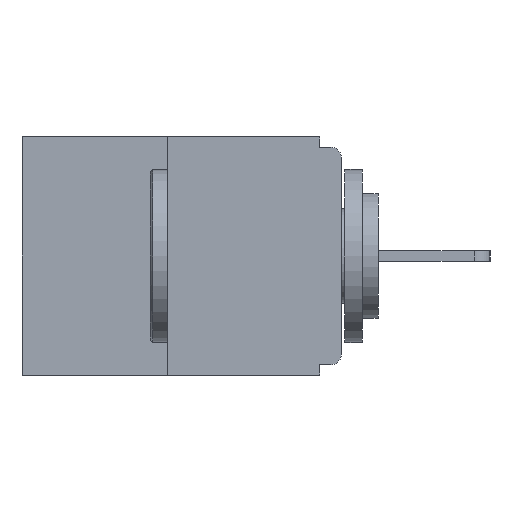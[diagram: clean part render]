
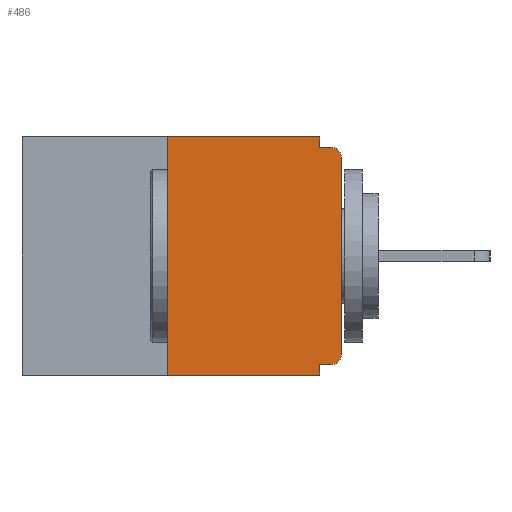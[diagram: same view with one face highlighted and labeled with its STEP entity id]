
A CAD part, left-side view. The second image highlights one B-rep face of the part: STEP entity #486.
In plain terms, the highlighted planar face has unit normal (-1, 0, 0).
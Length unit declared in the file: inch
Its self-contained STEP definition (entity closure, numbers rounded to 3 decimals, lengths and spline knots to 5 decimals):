
#286 = CARTESIAN_POINT ( 'NONE',  ( 0., 0., -0.313 ) ) ;
#466 = CARTESIAN_POINT ( 'NONE',  ( 0., 0.25, 0. ) ) ;
#486 = ADVANCED_FACE ( 'NONE', ( #17631 ), #12381, .F. ) ;
#744 = ORIENTED_EDGE ( 'NONE', *, *, #5234, .F. ) ;
#770 = DIRECTION ( 'NONE',  ( -1., 0., 0. ) ) ;
#903 = CIRCLE ( 'NONE', #10632, 0.015 ) ;
#1073 = VERTEX_POINT ( 'NONE', #5117 ) ;
#1312 = DIRECTION ( 'NONE',  ( 0., -1., 0. ) ) ;
#1439 = CARTESIAN_POINT ( 'NONE',  ( 0., 0.25, 0. ) ) ;
#2170 = EDGE_CURVE ( 'NONE', #10581, #12531, #15685, .T. ) ;
#2854 = CARTESIAN_POINT ( 'NONE',  ( 0., 0.015, -0.03 ) ) ;
#3157 = EDGE_CURVE ( 'NONE', #1073, #18803, #11619, .T. ) ;
#3238 = CIRCLE ( 'NONE', #18460, 0.015 ) ;
#3380 = VERTEX_POINT ( 'NONE', #466 ) ;
#3461 = EDGE_CURVE ( 'NONE', #7470, #10581, #3238, .T. ) ;
#3502 = CARTESIAN_POINT ( 'NONE',  ( 0., 0.46, 0. ) ) ;
#3644 = LINE ( 'NONE', #3765, #10192 ) ;
#3765 = CARTESIAN_POINT ( 'NONE',  ( 0., 0.031, -0.343 ) ) ;
#3949 = LINE ( 'NONE', #14905, #14942 ) ;
#4170 = DIRECTION ( 'NONE',  ( 0., -1., 0. ) ) ;
#4470 = CARTESIAN_POINT ( 'NONE',  ( 0., 0.25, -0.343 ) ) ;
#4524 = EDGE_CURVE ( 'NONE', #17603, #3380, #16032, .T. ) ;
#4822 = VECTOR ( 'NONE', #14132, 39.37008 ) ;
#5065 = DIRECTION ( 'NONE',  ( 0., 0., -1. ) ) ;
#5117 = CARTESIAN_POINT ( 'NONE',  ( 0., 0.031, 0. ) ) ;
#5234 = EDGE_CURVE ( 'NONE', #12884, #16886, #3644, .T. ) ;
#5411 = CARTESIAN_POINT ( 'NONE',  ( 0., 0.46, 0. ) ) ;
#5461 = CARTESIAN_POINT ( 'NONE',  ( 0., 0., 0. ) ) ;
#7470 = VERTEX_POINT ( 'NONE', #14377 ) ;
#7878 = LINE ( 'NONE', #7908, #18600 ) ;
#7908 = CARTESIAN_POINT ( 'NONE',  ( 0., 0., -0.328 ) ) ;
#8150 = CARTESIAN_POINT ( 'NONE',  ( 0., 0.015, -0.313 ) ) ;
#8322 = DIRECTION ( 'NONE',  ( 0., 0., 1. ) ) ;
#8785 = CARTESIAN_POINT ( 'NONE',  ( 0., 0.031, -0.328 ) ) ;
#8945 = DIRECTION ( 'NONE',  ( 0., 0., -1. ) ) ;
#9362 = EDGE_CURVE ( 'NONE', #17603, #16886, #16265, .T. ) ;
#10081 = CARTESIAN_POINT ( 'NONE',  ( 0., 0.031, -0.343 ) ) ;
#10192 = VECTOR ( 'NONE', #14229, 39.37008 ) ;
#10314 = DIRECTION ( 'NONE',  ( 0., 0., 1. ) ) ;
#10577 = ORIENTED_EDGE ( 'NONE', *, *, #3461, .T. ) ;
#10581 = VERTEX_POINT ( 'NONE', #286 ) ;
#10632 = AXIS2_PLACEMENT_3D ( 'NONE', #2854, #11844, #16499 ) ;
#10891 = VECTOR ( 'NONE', #4170, 39.37008 ) ;
#11148 = CARTESIAN_POINT ( 'NONE',  ( 0., 0., -0.03 ) ) ;
#11176 = ORIENTED_EDGE ( 'NONE', *, *, #19202, .F. ) ;
#11189 = DIRECTION ( 'NONE',  ( 0., 0., -1. ) ) ;
#11587 = ORIENTED_EDGE ( 'NONE', *, *, #3157, .F. ) ;
#11619 = LINE ( 'NONE', #13385, #13304 ) ;
#11681 = VECTOR ( 'NONE', #8322, 39.37008 ) ;
#11844 = DIRECTION ( 'NONE',  ( -1., 0., 0. ) ) ;
#12081 = EDGE_CURVE ( 'NONE', #12531, #16841, #903, .T. ) ;
#12381 = PLANE ( 'NONE',  #17246 ) ;
#12531 = VERTEX_POINT ( 'NONE', #11148 ) ;
#12812 = EDGE_CURVE ( 'NONE', #3380, #1073, #15372, .T. ) ;
#12884 = VERTEX_POINT ( 'NONE', #8785 ) ;
#12953 = ORIENTED_EDGE ( 'NONE', *, *, #4524, .F. ) ;
#13121 = CARTESIAN_POINT ( 'NONE',  ( 0., 0.015, -0.015 ) ) ;
#13304 = VECTOR ( 'NONE', #8945, 39.37008 ) ;
#13385 = CARTESIAN_POINT ( 'NONE',  ( 0., 0.031, 0. ) ) ;
#14132 = DIRECTION ( 'NONE',  ( 0., -1., 0. ) ) ;
#14229 = DIRECTION ( 'NONE',  ( 0., 0., -1. ) ) ;
#14377 = CARTESIAN_POINT ( 'NONE',  ( 0., 0.015, -0.328 ) ) ;
#14634 = VECTOR ( 'NONE', #10314, 39.37008 ) ;
#14905 = CARTESIAN_POINT ( 'NONE',  ( 0., 0., -0.015 ) ) ;
#14942 = VECTOR ( 'NONE', #1312, 39.37008 ) ;
#15265 = CARTESIAN_POINT ( 'NONE',  ( 0., 0.031, -0.015 ) ) ;
#15372 = LINE ( 'NONE', #5411, #10891 ) ;
#15473 = EDGE_LOOP ( 'NONE', ( #18954, #12953, #17836, #744, #11176, #10577, #15620, #17635, #17698, #11587 ) ) ;
#15620 = ORIENTED_EDGE ( 'NONE', *, *, #2170, .T. ) ;
#15685 = LINE ( 'NONE', #5461, #11681 ) ;
#16032 = LINE ( 'NONE', #1439, #14634 ) ;
#16167 = CARTESIAN_POINT ( 'NONE',  ( 0., 0.46, -0.343 ) ) ;
#16265 = LINE ( 'NONE', #16167, #4822 ) ;
#16499 = DIRECTION ( 'NONE',  ( 0., 0., -1. ) ) ;
#16841 = VERTEX_POINT ( 'NONE', #13121 ) ;
#16886 = VERTEX_POINT ( 'NONE', #10081 ) ;
#17246 = AXIS2_PLACEMENT_3D ( 'NONE', #3502, #18352, #5065 ) ;
#17603 = VERTEX_POINT ( 'NONE', #4470 ) ;
#17631 = FACE_OUTER_BOUND ( 'NONE', #15473, .T. ) ;
#17635 = ORIENTED_EDGE ( 'NONE', *, *, #12081, .T. ) ;
#17698 = ORIENTED_EDGE ( 'NONE', *, *, #18279, .F. ) ;
#17836 = ORIENTED_EDGE ( 'NONE', *, *, #9362, .T. ) ;
#18279 = EDGE_CURVE ( 'NONE', #18803, #16841, #3949, .T. ) ;
#18352 = DIRECTION ( 'NONE',  ( 1., 0., 0. ) ) ;
#18460 = AXIS2_PLACEMENT_3D ( 'NONE', #8150, #770, #11189 ) ;
#18563 = DIRECTION ( 'NONE',  ( 0., 1., 0. ) ) ;
#18600 = VECTOR ( 'NONE', #18563, 39.37008 ) ;
#18803 = VERTEX_POINT ( 'NONE', #15265 ) ;
#18954 = ORIENTED_EDGE ( 'NONE', *, *, #12812, .F. ) ;
#19202 = EDGE_CURVE ( 'NONE', #7470, #12884, #7878, .T. ) ;
